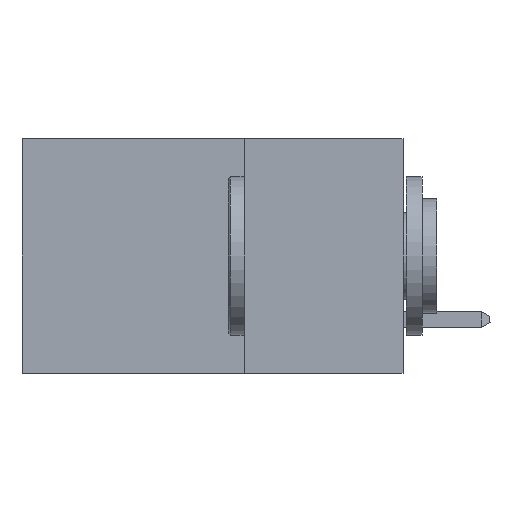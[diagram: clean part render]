
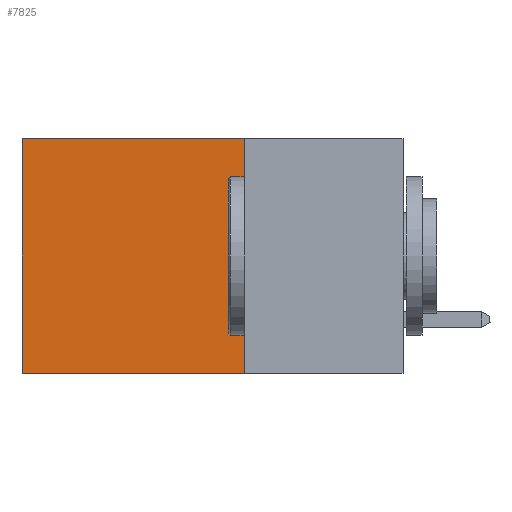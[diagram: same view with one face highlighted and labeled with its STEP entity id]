
A CAD part, left-side view. The second image highlights one B-rep face of the part: STEP entity #7825.
In plain terms, the highlighted planar face has unit normal (-1, 0, 0).
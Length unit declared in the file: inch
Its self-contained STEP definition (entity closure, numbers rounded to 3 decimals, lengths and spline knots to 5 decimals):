
#14 = VECTOR ( 'NONE', #7811, 39.37008 ) ;
#135 = CARTESIAN_POINT ( 'NONE',  ( 0.2875, 0.25, -0.37 ) ) ;
#557 = FACE_OUTER_BOUND ( 'NONE', #8720, .T. ) ;
#854 = CARTESIAN_POINT ( 'NONE',  ( 0.2875, 0.25, 0. ) ) ;
#1613 = ORIENTED_EDGE ( 'NONE', *, *, #2672, .F. ) ;
#2004 = EDGE_CURVE ( 'NONE', #10782, #8258, #4472, .T. ) ;
#2337 = VECTOR ( 'NONE', #3443, 39.37008 ) ;
#2544 = ORIENTED_EDGE ( 'NONE', *, *, #8060, .F. ) ;
#2664 = VECTOR ( 'NONE', #9231, 39.37008 ) ;
#2672 = EDGE_CURVE ( 'NONE', #4813, #8258, #6414, .T. ) ;
#3329 = CARTESIAN_POINT ( 'NONE',  ( 0.2875, 0.6, 0. ) ) ;
#3443 = DIRECTION ( 'NONE',  ( 0., 1., 0. ) ) ;
#4018 = ORIENTED_EDGE ( 'NONE', *, *, #11544, .T. ) ;
#4086 = ORIENTED_EDGE ( 'NONE', *, *, #2004, .T. ) ;
#4472 = LINE ( 'NONE', #3329, #12436 ) ;
#4623 = CARTESIAN_POINT ( 'NONE',  ( 0.2875, 0.6, 0. ) ) ;
#4707 = VERTEX_POINT ( 'NONE', #12509 ) ;
#4813 = VERTEX_POINT ( 'NONE', #135 ) ;
#6414 = LINE ( 'NONE', #9827, #14 ) ;
#7811 = DIRECTION ( 'NONE',  ( 0., 1., 0. ) ) ;
#7825 = ADVANCED_FACE ( 'NONE', ( #557 ), #8665, .F. ) ;
#8060 = EDGE_CURVE ( 'NONE', #4707, #4813, #10394, .T. ) ;
#8258 = VERTEX_POINT ( 'NONE', #11952 ) ;
#8315 = CARTESIAN_POINT ( 'NONE',  ( 0.2875, 0.25, 0. ) ) ;
#8665 = PLANE ( 'NONE',  #11692 ) ;
#8710 = DIRECTION ( 'NONE',  ( 0., 0., -1. ) ) ;
#8720 = EDGE_LOOP ( 'NONE', ( #4086, #1613, #2544, #4018 ) ) ;
#9231 = DIRECTION ( 'NONE',  ( 0., 0., -1. ) ) ;
#9827 = CARTESIAN_POINT ( 'NONE',  ( 0.2875, 0.25, -0.37 ) ) ;
#10122 = DIRECTION ( 'NONE',  ( 0., 0., -1. ) ) ;
#10394 = LINE ( 'NONE', #12053, #2664 ) ;
#10782 = VERTEX_POINT ( 'NONE', #4623 ) ;
#11498 = DIRECTION ( 'NONE',  ( 1., 0., 0. ) ) ;
#11544 = EDGE_CURVE ( 'NONE', #4707, #10782, #11845, .T. ) ;
#11692 = AXIS2_PLACEMENT_3D ( 'NONE', #854, #11498, #8710 ) ;
#11845 = LINE ( 'NONE', #8315, #2337 ) ;
#11952 = CARTESIAN_POINT ( 'NONE',  ( 0.2875, 0.6, -0.37 ) ) ;
#12053 = CARTESIAN_POINT ( 'NONE',  ( 0.2875, 0.25, 0. ) ) ;
#12436 = VECTOR ( 'NONE', #10122, 39.37008 ) ;
#12509 = CARTESIAN_POINT ( 'NONE',  ( 0.2875, 0.25, 0. ) ) ;
